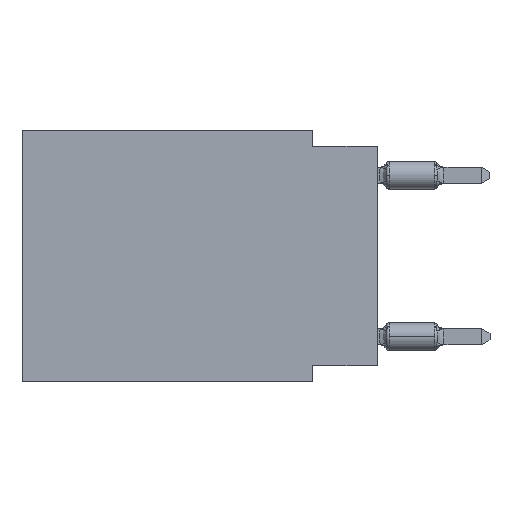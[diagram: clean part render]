
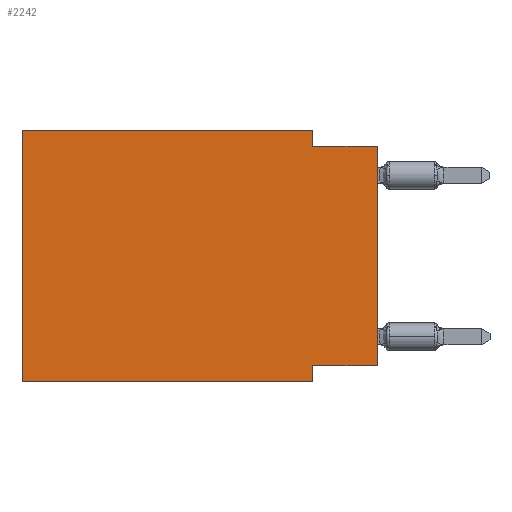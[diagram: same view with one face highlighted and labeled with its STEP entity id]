
A CAD part, left-side view. The second image highlights one B-rep face of the part: STEP entity #2242.
In plain terms, the highlighted planar face has unit normal (-1, 0, 0).
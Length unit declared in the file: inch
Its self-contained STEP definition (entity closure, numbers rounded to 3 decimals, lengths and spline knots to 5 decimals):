
#221 = LINE ( 'NONE', #9122, #18543 ) ;
#903 = CARTESIAN_POINT ( 'NONE',  ( 0., 0.1, 0. ) ) ;
#1054 = LINE ( 'NONE', #12527, #11846 ) ;
#1338 = LINE ( 'NONE', #12246, #10757 ) ;
#1406 = ORIENTED_EDGE ( 'NONE', *, *, #18117, .F. ) ;
#1668 = ORIENTED_EDGE ( 'NONE', *, *, #13275, .T. ) ;
#1719 = ORIENTED_EDGE ( 'NONE', *, *, #14038, .F. ) ;
#1845 = VECTOR ( 'NONE', #14059, 39.37008 ) ;
#2227 = VECTOR ( 'NONE', #2285, 39.37008 ) ;
#2242 = ADVANCED_FACE ( 'NONE', ( #2413 ), #16696, .F. ) ;
#2285 = DIRECTION ( 'NONE',  ( 0., 0., 1. ) ) ;
#2413 = FACE_OUTER_BOUND ( 'NONE', #17173, .T. ) ;
#2699 = DIRECTION ( 'NONE',  ( 0., 0., -1. ) ) ;
#3747 = VECTOR ( 'NONE', #3903, 39.37008 ) ;
#3903 = DIRECTION ( 'NONE',  ( 0., -1., 0. ) ) ;
#3996 = DIRECTION ( 'NONE',  ( 0., 0., -1. ) ) ;
#4128 = EDGE_CURVE ( 'NONE', #15871, #8275, #13787, .T. ) ;
#4250 = CARTESIAN_POINT ( 'NONE',  ( 0., 0.1, -0.365 ) ) ;
#4255 = CARTESIAN_POINT ( 'NONE',  ( 0., 0.1, -0.025 ) ) ;
#5415 = CARTESIAN_POINT ( 'NONE',  ( 0., 0.1, 0. ) ) ;
#6526 = LINE ( 'NONE', #12274, #2227 ) ;
#6736 = DIRECTION ( 'NONE',  ( 1., 0., 0. ) ) ;
#6775 = DIRECTION ( 'NONE',  ( 0., -1., 0. ) ) ;
#6932 = VERTEX_POINT ( 'NONE', #4250 ) ;
#6976 = EDGE_CURVE ( 'NONE', #7049, #13287, #1338, .T. ) ;
#7049 = VERTEX_POINT ( 'NONE', #9313 ) ;
#7500 = CARTESIAN_POINT ( 'NONE',  ( 0., 0.1, -0.39 ) ) ;
#8275 = VERTEX_POINT ( 'NONE', #4255 ) ;
#8304 = CARTESIAN_POINT ( 'NONE',  ( 0., 0.55, 0. ) ) ;
#9122 = CARTESIAN_POINT ( 'NONE',  ( 0., 0., -0.365 ) ) ;
#9185 = CARTESIAN_POINT ( 'NONE',  ( 0., 0.1, -0.39 ) ) ;
#9313 = CARTESIAN_POINT ( 'NONE',  ( 0., 0., -0.365 ) ) ;
#9617 = VERTEX_POINT ( 'NONE', #10490 ) ;
#9814 = CARTESIAN_POINT ( 'NONE',  ( 0., 0., -0.025 ) ) ;
#9938 = EDGE_CURVE ( 'NONE', #10826, #15871, #15450, .T. ) ;
#10482 = ORIENTED_EDGE ( 'NONE', *, *, #4128, .F. ) ;
#10490 = CARTESIAN_POINT ( 'NONE',  ( 0., 0.55, -0.39 ) ) ;
#10542 = DIRECTION ( 'NONE',  ( 0., 1., 0. ) ) ;
#10642 = DIRECTION ( 'NONE',  ( 0., 0., 1. ) ) ;
#10757 = VECTOR ( 'NONE', #10642, 39.37008 ) ;
#10826 = VERTEX_POINT ( 'NONE', #11457 ) ;
#10954 = LINE ( 'NONE', #9814, #3747 ) ;
#11085 = ORIENTED_EDGE ( 'NONE', *, *, #13405, .F. ) ;
#11093 = ORIENTED_EDGE ( 'NONE', *, *, #9938, .F. ) ;
#11125 = CARTESIAN_POINT ( 'NONE',  ( 0., 0., -0.025 ) ) ;
#11339 = VECTOR ( 'NONE', #3996, 39.37008 ) ;
#11457 = CARTESIAN_POINT ( 'NONE',  ( 0., 0.55, 0. ) ) ;
#11846 = VECTOR ( 'NONE', #6775, 39.37008 ) ;
#12225 = VERTEX_POINT ( 'NONE', #7500 ) ;
#12246 = CARTESIAN_POINT ( 'NONE',  ( 0., 0., 0. ) ) ;
#12274 = CARTESIAN_POINT ( 'NONE',  ( 0., 0.55, 0. ) ) ;
#12455 = ORIENTED_EDGE ( 'NONE', *, *, #12853, .F. ) ;
#12527 = CARTESIAN_POINT ( 'NONE',  ( 0., 0.55, -0.39 ) ) ;
#12853 = EDGE_CURVE ( 'NONE', #9617, #10826, #6526, .T. ) ;
#13157 = DIRECTION ( 'NONE',  ( 0., 0., -1. ) ) ;
#13275 = EDGE_CURVE ( 'NONE', #9617, #12225, #1054, .T. ) ;
#13287 = VERTEX_POINT ( 'NONE', #11125 ) ;
#13405 = EDGE_CURVE ( 'NONE', #6932, #12225, #17655, .T. ) ;
#13787 = LINE ( 'NONE', #903, #11339 ) ;
#14038 = EDGE_CURVE ( 'NONE', #8275, #13287, #10954, .T. ) ;
#14059 = DIRECTION ( 'NONE',  ( 0., -1., 0. ) ) ;
#14568 = VECTOR ( 'NONE', #13157, 39.37008 ) ;
#14578 = AXIS2_PLACEMENT_3D ( 'NONE', #16796, #6736, #2699 ) ;
#15450 = LINE ( 'NONE', #8304, #1845 ) ;
#15871 = VERTEX_POINT ( 'NONE', #5415 ) ;
#16696 = PLANE ( 'NONE',  #14578 ) ;
#16796 = CARTESIAN_POINT ( 'NONE',  ( 0., 0.55, 0. ) ) ;
#17173 = EDGE_LOOP ( 'NONE', ( #17648, #1719, #10482, #11093, #12455, #1668, #11085, #1406 ) ) ;
#17648 = ORIENTED_EDGE ( 'NONE', *, *, #6976, .T. ) ;
#17655 = LINE ( 'NONE', #9185, #14568 ) ;
#18117 = EDGE_CURVE ( 'NONE', #7049, #6932, #221, .T. ) ;
#18543 = VECTOR ( 'NONE', #10542, 39.37008 ) ;
